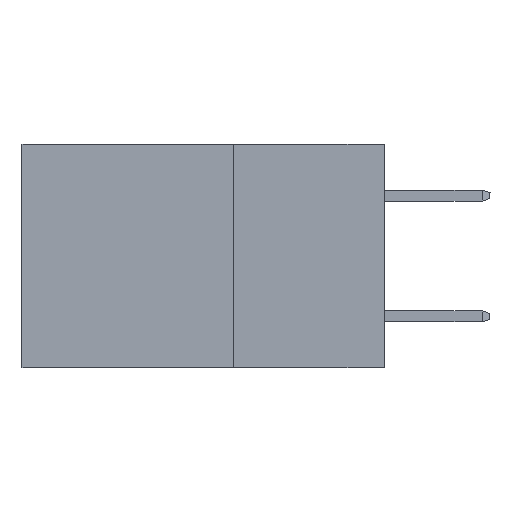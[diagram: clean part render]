
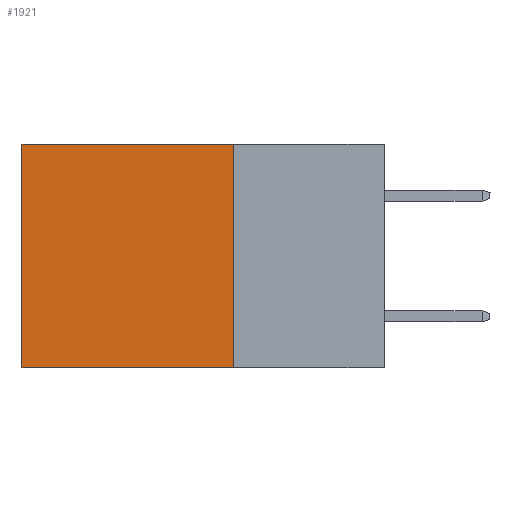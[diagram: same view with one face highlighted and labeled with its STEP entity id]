
A CAD part, left-side view. The second image highlights one B-rep face of the part: STEP entity #1921.
In plain terms, the highlighted planar face has unit normal (-1, 0, 0).
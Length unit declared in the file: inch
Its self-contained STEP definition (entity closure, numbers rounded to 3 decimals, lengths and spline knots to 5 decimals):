
#517 = EDGE_CURVE ( 'NONE', #1235, #4995, #9702, .T. ) ;
#755 = DIRECTION ( 'NONE',  ( 0., 0., -1. ) ) ;
#877 = VECTOR ( 'NONE', #4519, 39.37008 ) ;
#1060 = VECTOR ( 'NONE', #5801, 39.37008 ) ;
#1235 = VERTEX_POINT ( 'NONE', #4569 ) ;
#1921 = ADVANCED_FACE ( 'NONE', ( #5229 ), #7054, .F. ) ;
#2368 = ORIENTED_EDGE ( 'NONE', *, *, #517, .T. ) ;
#2619 = CARTESIAN_POINT ( 'NONE',  ( 0.298, 0.25, 0. ) ) ;
#3019 = EDGE_LOOP ( 'NONE', ( #2368, #7095, #9167, #5552 ) ) ;
#3695 = DIRECTION ( 'NONE',  ( 0., 0., -1. ) ) ;
#3780 = CARTESIAN_POINT ( 'NONE',  ( 0.298, 0.25, 0. ) ) ;
#4071 = EDGE_CURVE ( 'NONE', #8541, #8659, #8969, .T. ) ;
#4450 = CARTESIAN_POINT ( 'NONE',  ( 0.298, 0.6, 0. ) ) ;
#4519 = DIRECTION ( 'NONE',  ( 0., 1., 0. ) ) ;
#4569 = CARTESIAN_POINT ( 'NONE',  ( 0.298, 0.6, 0. ) ) ;
#4663 = DIRECTION ( 'NONE',  ( 0., 1., 0. ) ) ;
#4936 = EDGE_CURVE ( 'NONE', #8541, #1235, #6754, .T. ) ;
#4995 = VERTEX_POINT ( 'NONE', #7729 ) ;
#5136 = CARTESIAN_POINT ( 'NONE',  ( 0.298, 0.25, 0. ) ) ;
#5229 = FACE_OUTER_BOUND ( 'NONE', #3019, .T. ) ;
#5546 = AXIS2_PLACEMENT_3D ( 'NONE', #6234, #6988, #755 ) ;
#5552 = ORIENTED_EDGE ( 'NONE', *, *, #4936, .T. ) ;
#5801 = DIRECTION ( 'NONE',  ( 0., 0., -1. ) ) ;
#6026 = CARTESIAN_POINT ( 'NONE',  ( 0.298, 0.25, -0.37 ) ) ;
#6144 = CARTESIAN_POINT ( 'NONE',  ( 0.298, 0.25, -0.37 ) ) ;
#6234 = CARTESIAN_POINT ( 'NONE',  ( 0.298, 0.25, 0. ) ) ;
#6754 = LINE ( 'NONE', #3780, #8957 ) ;
#6988 = DIRECTION ( 'NONE',  ( 1., 0., 0. ) ) ;
#7054 = PLANE ( 'NONE',  #5546 ) ;
#7095 = ORIENTED_EDGE ( 'NONE', *, *, #8199, .F. ) ;
#7729 = CARTESIAN_POINT ( 'NONE',  ( 0.298, 0.6, -0.37 ) ) ;
#8199 = EDGE_CURVE ( 'NONE', #8659, #4995, #9727, .T. ) ;
#8541 = VERTEX_POINT ( 'NONE', #2619 ) ;
#8659 = VERTEX_POINT ( 'NONE', #6144 ) ;
#8957 = VECTOR ( 'NONE', #4663, 39.37008 ) ;
#8969 = LINE ( 'NONE', #5136, #1060 ) ;
#9167 = ORIENTED_EDGE ( 'NONE', *, *, #4071, .F. ) ;
#9702 = LINE ( 'NONE', #4450, #9818 ) ;
#9727 = LINE ( 'NONE', #6026, #877 ) ;
#9818 = VECTOR ( 'NONE', #3695, 39.37008 ) ;
